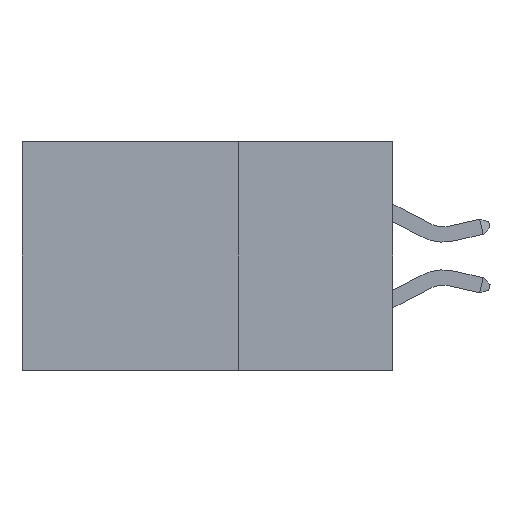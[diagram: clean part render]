
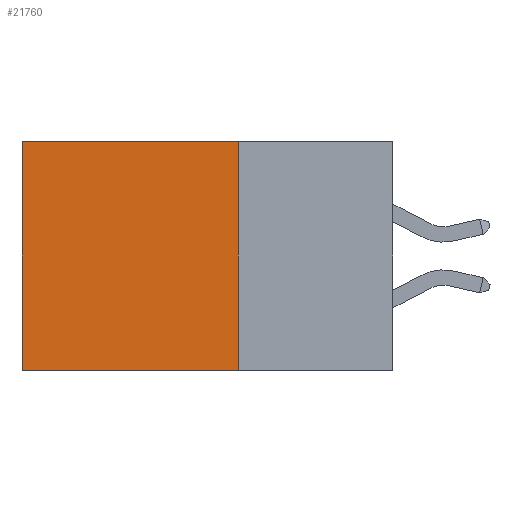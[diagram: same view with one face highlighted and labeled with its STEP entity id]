
A CAD part, left-side view. The second image highlights one B-rep face of the part: STEP entity #21760.
In plain terms, the highlighted planar face has unit normal (-1, 0, 0).
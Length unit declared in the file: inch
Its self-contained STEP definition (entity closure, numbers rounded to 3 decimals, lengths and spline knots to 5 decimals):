
#343 = LINE ( 'NONE', #1166, #4567 ) ;
#1019 = CARTESIAN_POINT ( 'NONE',  ( 0.2875, 0.25, 0. ) ) ;
#1166 = CARTESIAN_POINT ( 'NONE',  ( 0.2875, 0.25, -0.37 ) ) ;
#1398 = CARTESIAN_POINT ( 'NONE',  ( 0.2875, 0.6, 0. ) ) ;
#2828 = DIRECTION ( 'NONE',  ( 0., 0., -1. ) ) ;
#2972 = ORIENTED_EDGE ( 'NONE', *, *, #12188, .T. ) ;
#3052 = CARTESIAN_POINT ( 'NONE',  ( 0.2875, 0.6, -0.37 ) ) ;
#4268 = ORIENTED_EDGE ( 'NONE', *, *, #16795, .F. ) ;
#4393 = VERTEX_POINT ( 'NONE', #7321 ) ;
#4567 = VECTOR ( 'NONE', #13767, 39.37008 ) ;
#4571 = PLANE ( 'NONE',  #20487 ) ;
#4652 = VECTOR ( 'NONE', #10404, 39.37008 ) ;
#6901 = EDGE_LOOP ( 'NONE', ( #18400, #4268, #7432, #2972 ) ) ;
#7321 = CARTESIAN_POINT ( 'NONE',  ( 0.2875, 0.25, 0. ) ) ;
#7432 = ORIENTED_EDGE ( 'NONE', *, *, #15914, .F. ) ;
#7437 = VERTEX_POINT ( 'NONE', #3052 ) ;
#8023 = VERTEX_POINT ( 'NONE', #17625 ) ;
#8486 = VECTOR ( 'NONE', #16407, 39.37008 ) ;
#8654 = CARTESIAN_POINT ( 'NONE',  ( 0.2875, 0.25, -0.37 ) ) ;
#8898 = FACE_OUTER_BOUND ( 'NONE', #6901, .T. ) ;
#9040 = LINE ( 'NONE', #12777, #8486 ) ;
#10203 = DIRECTION ( 'NONE',  ( 0., 1., 0. ) ) ;
#10404 = DIRECTION ( 'NONE',  ( 0., 0., -1. ) ) ;
#10518 = VECTOR ( 'NONE', #10203, 39.37008 ) ;
#10741 = EDGE_CURVE ( 'NONE', #8023, #7437, #19018, .T. ) ;
#12188 = EDGE_CURVE ( 'NONE', #4393, #8023, #20067, .T. ) ;
#12777 = CARTESIAN_POINT ( 'NONE',  ( 0.2875, 0.25, 0. ) ) ;
#13615 = DIRECTION ( 'NONE',  ( 1., 0., 0. ) ) ;
#13767 = DIRECTION ( 'NONE',  ( 0., 1., 0. ) ) ;
#14852 = VERTEX_POINT ( 'NONE', #8654 ) ;
#15562 = CARTESIAN_POINT ( 'NONE',  ( 0.2875, 0.25, 0. ) ) ;
#15914 = EDGE_CURVE ( 'NONE', #4393, #14852, #9040, .T. ) ;
#16407 = DIRECTION ( 'NONE',  ( 0., 0., -1. ) ) ;
#16795 = EDGE_CURVE ( 'NONE', #14852, #7437, #343, .T. ) ;
#17625 = CARTESIAN_POINT ( 'NONE',  ( 0.2875, 0.6, 0. ) ) ;
#18400 = ORIENTED_EDGE ( 'NONE', *, *, #10741, .T. ) ;
#19018 = LINE ( 'NONE', #1398, #4652 ) ;
#20067 = LINE ( 'NONE', #15562, #10518 ) ;
#20487 = AXIS2_PLACEMENT_3D ( 'NONE', #1019, #13615, #2828 ) ;
#21760 = ADVANCED_FACE ( 'NONE', ( #8898 ), #4571, .F. ) ;
